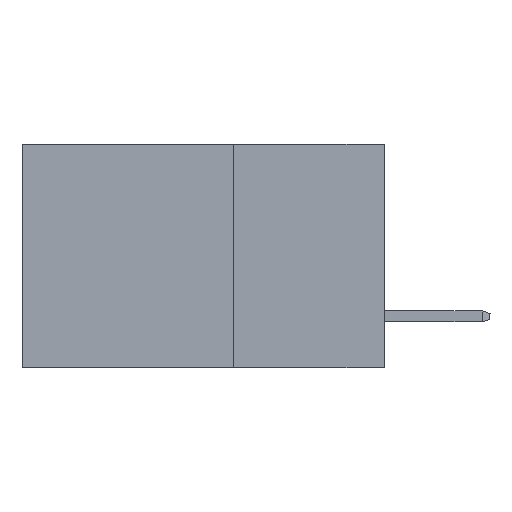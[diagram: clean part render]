
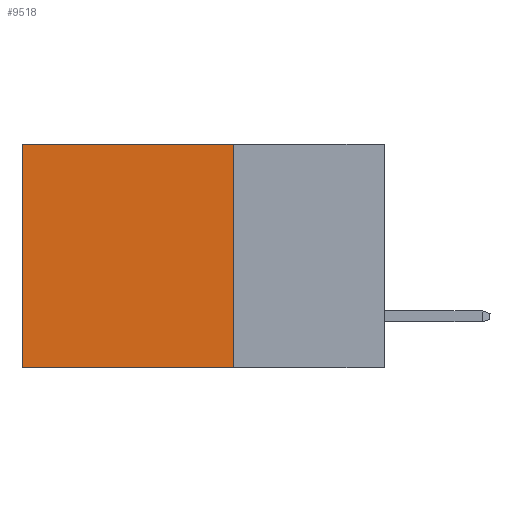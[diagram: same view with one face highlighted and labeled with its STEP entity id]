
A CAD part, left-side view. The second image highlights one B-rep face of the part: STEP entity #9518.
In plain terms, the highlighted planar face has unit normal (-1, 0, 0).
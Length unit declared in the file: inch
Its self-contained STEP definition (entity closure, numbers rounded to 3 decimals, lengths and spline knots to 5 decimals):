
#69 = AXIS2_PLACEMENT_3D ( 'NONE', #7672, #17589, #16300 ) ;
#605 = CARTESIAN_POINT ( 'NONE',  ( 0.298, 0.25, 0. ) ) ;
#766 = CARTESIAN_POINT ( 'NONE',  ( 0.298, 0.6, 0. ) ) ;
#2170 = VERTEX_POINT ( 'NONE', #12136 ) ;
#2705 = VERTEX_POINT ( 'NONE', #9680 ) ;
#3227 = VECTOR ( 'NONE', #7748, 39.37008 ) ;
#4015 = CARTESIAN_POINT ( 'NONE',  ( 0.298, 0.25, -0.37 ) ) ;
#4441 = EDGE_CURVE ( 'NONE', #2705, #16134, #9822, .T. ) ;
#5665 = LINE ( 'NONE', #605, #14471 ) ;
#6450 = CARTESIAN_POINT ( 'NONE',  ( 0.298, 0.25, 0. ) ) ;
#7262 = ORIENTED_EDGE ( 'NONE', *, *, #11749, .F. ) ;
#7497 = PLANE ( 'NONE',  #69 ) ;
#7533 = CARTESIAN_POINT ( 'NONE',  ( 0.298, 0.25, -0.37 ) ) ;
#7606 = VERTEX_POINT ( 'NONE', #12657 ) ;
#7672 = CARTESIAN_POINT ( 'NONE',  ( 0.298, 0.25, 0. ) ) ;
#7748 = DIRECTION ( 'NONE',  ( 0., 0., -1. ) ) ;
#7811 = EDGE_CURVE ( 'NONE', #2170, #7606, #10335, .T. ) ;
#8318 = FACE_OUTER_BOUND ( 'NONE', #17224, .T. ) ;
#9518 = ADVANCED_FACE ( 'NONE', ( #8318 ), #7497, .F. ) ;
#9680 = CARTESIAN_POINT ( 'NONE',  ( 0.298, 0.25, 0. ) ) ;
#9821 = LINE ( 'NONE', #7533, #16722 ) ;
#9822 = LINE ( 'NONE', #6450, #11961 ) ;
#10161 = ORIENTED_EDGE ( 'NONE', *, *, #4441, .F. ) ;
#10335 = LINE ( 'NONE', #766, #3227 ) ;
#10674 = DIRECTION ( 'NONE',  ( 0., 0., -1. ) ) ;
#10768 = ORIENTED_EDGE ( 'NONE', *, *, #7811, .T. ) ;
#11501 = DIRECTION ( 'NONE',  ( 0., 1., 0. ) ) ;
#11749 = EDGE_CURVE ( 'NONE', #16134, #7606, #9821, .T. ) ;
#11961 = VECTOR ( 'NONE', #10674, 39.37008 ) ;
#12136 = CARTESIAN_POINT ( 'NONE',  ( 0.298, 0.6, 0. ) ) ;
#12657 = CARTESIAN_POINT ( 'NONE',  ( 0.298, 0.6, -0.37 ) ) ;
#14359 = EDGE_CURVE ( 'NONE', #2705, #2170, #5665, .T. ) ;
#14471 = VECTOR ( 'NONE', #11501, 39.37008 ) ;
#15783 = ORIENTED_EDGE ( 'NONE', *, *, #14359, .T. ) ;
#16134 = VERTEX_POINT ( 'NONE', #4015 ) ;
#16300 = DIRECTION ( 'NONE',  ( 0., 0., -1. ) ) ;
#16722 = VECTOR ( 'NONE', #17057, 39.37008 ) ;
#17057 = DIRECTION ( 'NONE',  ( 0., 1., 0. ) ) ;
#17224 = EDGE_LOOP ( 'NONE', ( #10768, #7262, #10161, #15783 ) ) ;
#17589 = DIRECTION ( 'NONE',  ( 1., 0., 0. ) ) ;
